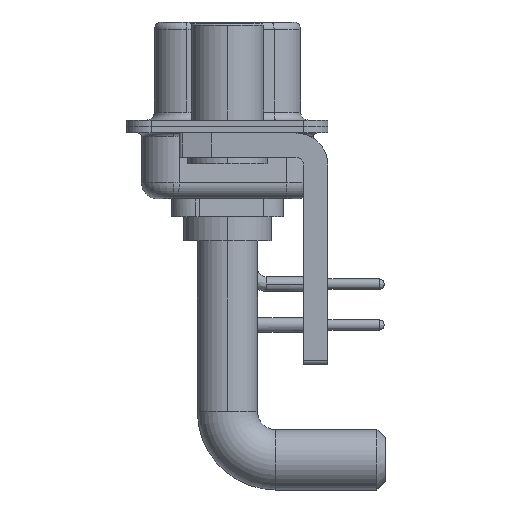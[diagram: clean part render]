
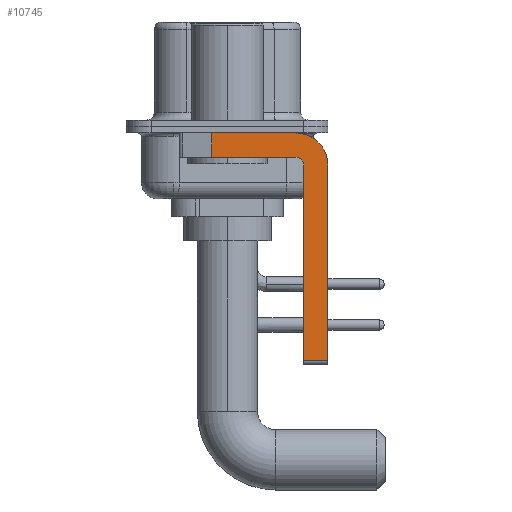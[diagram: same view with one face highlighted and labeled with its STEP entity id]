
A CAD part, left-side view. The second image highlights one B-rep face of the part: STEP entity #10745.
In plain terms, the highlighted planar face has unit normal (-1, 0, 0).
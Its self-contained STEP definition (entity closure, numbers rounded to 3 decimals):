
#6 = EDGE_CURVE ( 'NONE', #8928, #3636, #28649, .T. ) ;
#38 = ORIENTED_EDGE ( 'NONE', *, *, #12410, .F. ) ;
#87 = DIRECTION ( 'NONE',  ( 0., 0., 1. ) ) ;
#849 = CARTESIAN_POINT ( 'NONE',  ( -2.9, -4.25, -0.4 ) ) ;
#1309 = DIRECTION ( 'NONE',  ( 0., -1., 0. ) ) ;
#1496 = CARTESIAN_POINT ( 'NONE',  ( -2.9, -4.25, -1.9 ) ) ;
#1720 = EDGE_CURVE ( 'NONE', #7018, #17834, #18593, .T. ) ;
#1754 = VECTOR ( 'NONE', #87, 1000. ) ;
#2337 = CARTESIAN_POINT ( 'NONE',  ( -2.9, -6.25, -2.4 ) ) ;
#2635 = LINE ( 'NONE', #24058, #24447 ) ;
#3035 = CARTESIAN_POINT ( 'NONE',  ( -2.9, -6.25, -2.4 ) ) ;
#3087 = EDGE_CURVE ( 'NONE', #19427, #15126, #13022, .T. ) ;
#3636 = VERTEX_POINT ( 'NONE', #2337 ) ;
#3689 = DIRECTION ( 'NONE',  ( 0., -1., 0. ) ) ;
#3977 = EDGE_CURVE ( 'NONE', #7018, #8928, #13093, .T. ) ;
#4263 = CARTESIAN_POINT ( 'NONE',  ( -2.9, 3., -0.4 ) ) ;
#4803 = VECTOR ( 'NONE', #26147, 1000. ) ;
#4944 = ORIENTED_EDGE ( 'NONE', *, *, #14903, .F. ) ;
#5033 = CARTESIAN_POINT ( 'NONE',  ( -2.9, -4.75, -14.8 ) ) ;
#5202 = ORIENTED_EDGE ( 'NONE', *, *, #3977, .F. ) ;
#5913 = DIRECTION ( 'NONE',  ( 0., 0., -1. ) ) ;
#7018 = VERTEX_POINT ( 'NONE', #25249 ) ;
#7176 = DIRECTION ( 'NONE',  ( 0., 0., -1. ) ) ;
#7416 = CARTESIAN_POINT ( 'NONE',  ( -2.9, -4.25, -2.4 ) ) ;
#7666 = AXIS2_PLACEMENT_3D ( 'NONE', #21940, #10390, #5913 ) ;
#8217 = FACE_OUTER_BOUND ( 'NONE', #14042, .T. ) ;
#8928 = VERTEX_POINT ( 'NONE', #849 ) ;
#9386 = ORIENTED_EDGE ( 'NONE', *, *, #21739, .F. ) ;
#10390 = DIRECTION ( 'NONE',  ( 1., 0., 0. ) ) ;
#10745 = ADVANCED_FACE ( 'NONE', ( #8217 ), #15609, .F. ) ;
#10984 = CARTESIAN_POINT ( 'NONE',  ( -2.9, 0.978, -1.9 ) ) ;
#11808 = LINE ( 'NONE', #5033, #1754 ) ;
#11879 = VERTEX_POINT ( 'NONE', #16207 ) ;
#12410 = EDGE_CURVE ( 'NONE', #3636, #15126, #21365, .T. ) ;
#13022 = LINE ( 'NONE', #22411, #29230 ) ;
#13093 = LINE ( 'NONE', #4263, #15452 ) ;
#14042 = EDGE_LOOP ( 'NONE', ( #5202, #28584, #9386, #18002, #4944, #26329, #38, #24134 ) ) ;
#14267 = CARTESIAN_POINT ( 'NONE',  ( -2.9, 0.978, -1.9 ) ) ;
#14903 = EDGE_CURVE ( 'NONE', #19427, #11879, #11808, .T. ) ;
#15126 = VERTEX_POINT ( 'NONE', #28552 ) ;
#15452 = VECTOR ( 'NONE', #3689, 1000. ) ;
#15609 = PLANE ( 'NONE',  #7666 ) ;
#16207 = CARTESIAN_POINT ( 'NONE',  ( -2.9, -4.75, -2.4 ) ) ;
#16347 = DIRECTION ( 'NONE',  ( 0., 1., 0. ) ) ;
#17070 = EDGE_CURVE ( 'NONE', #11879, #27327, #25971, .T. ) ;
#17834 = VERTEX_POINT ( 'NONE', #10984 ) ;
#18002 = ORIENTED_EDGE ( 'NONE', *, *, #17070, .F. ) ;
#18593 = LINE ( 'NONE', #14267, #25632 ) ;
#19067 = CARTESIAN_POINT ( 'NONE',  ( -2.9, -4.25, -2.4 ) ) ;
#19333 = AXIS2_PLACEMENT_3D ( 'NONE', #19067, #28447, #19820 ) ;
#19427 = VERTEX_POINT ( 'NONE', #19567 ) ;
#19567 = CARTESIAN_POINT ( 'NONE',  ( -2.9, -4.75, -14.55 ) ) ;
#19820 = DIRECTION ( 'NONE',  ( 0., 0., -1. ) ) ;
#21365 = LINE ( 'NONE', #3035, #4803 ) ;
#21602 = DIRECTION ( 'NONE',  ( -1., 0., 0. ) ) ;
#21739 = EDGE_CURVE ( 'NONE', #27327, #17834, #2635, .T. ) ;
#21940 = CARTESIAN_POINT ( 'NONE',  ( -2.9, -4.25, -2.4 ) ) ;
#22411 = CARTESIAN_POINT ( 'NONE',  ( -2.9, -4.25, -14.55 ) ) ;
#23999 = AXIS2_PLACEMENT_3D ( 'NONE', #7416, #21602, #26814 ) ;
#24058 = CARTESIAN_POINT ( 'NONE',  ( -2.9, -4.25, -1.9 ) ) ;
#24134 = ORIENTED_EDGE ( 'NONE', *, *, #6, .F. ) ;
#24447 = VECTOR ( 'NONE', #16347, 1000. ) ;
#25249 = CARTESIAN_POINT ( 'NONE',  ( -2.9, 0.978, -0.4 ) ) ;
#25632 = VECTOR ( 'NONE', #7176, 1000. ) ;
#25971 = CIRCLE ( 'NONE', #23999, 0.5 ) ;
#26147 = DIRECTION ( 'NONE',  ( 0., 0., -1. ) ) ;
#26329 = ORIENTED_EDGE ( 'NONE', *, *, #3087, .T. ) ;
#26814 = DIRECTION ( 'NONE',  ( 0., 0., 1. ) ) ;
#27327 = VERTEX_POINT ( 'NONE', #1496 ) ;
#28447 = DIRECTION ( 'NONE',  ( 1., 0., 0. ) ) ;
#28552 = CARTESIAN_POINT ( 'NONE',  ( -2.9, -6.25, -14.55 ) ) ;
#28584 = ORIENTED_EDGE ( 'NONE', *, *, #1720, .T. ) ;
#28649 = CIRCLE ( 'NONE', #19333, 2. ) ;
#29230 = VECTOR ( 'NONE', #1309, 1000. ) ;
